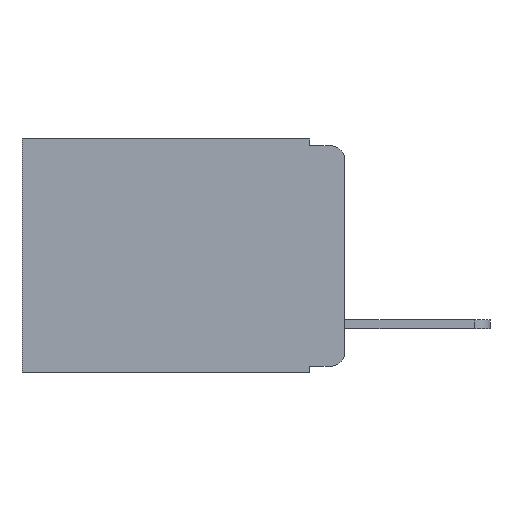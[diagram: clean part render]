
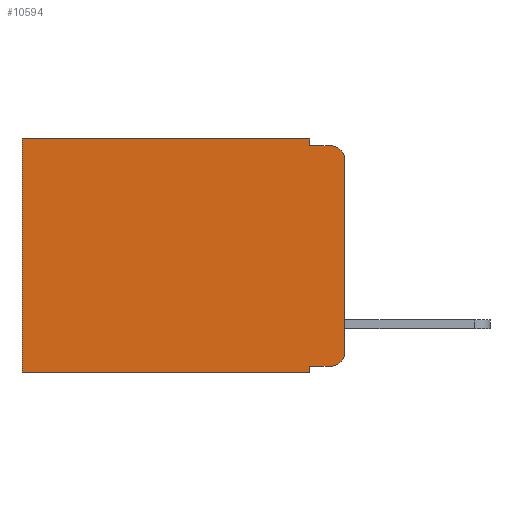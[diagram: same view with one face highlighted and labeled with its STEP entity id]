
A CAD part, left-side view. The second image highlights one B-rep face of the part: STEP entity #10594.
In plain terms, the highlighted planar face has unit normal (-1, 0, 0).
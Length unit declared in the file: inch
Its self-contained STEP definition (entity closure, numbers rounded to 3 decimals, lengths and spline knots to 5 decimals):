
#261 = AXIS2_PLACEMENT_3D ( 'NONE', #12687, #14218, #4974 ) ;
#318 = ORIENTED_EDGE ( 'NONE', *, *, #17588, .T. ) ;
#706 = DIRECTION ( 'NONE',  ( 0., 0., -1. ) ) ;
#741 = CARTESIAN_POINT ( 'NONE',  ( 0.298, 0., 0. ) ) ;
#1103 = VECTOR ( 'NONE', #18424, 39.37008 ) ;
#1160 = ORIENTED_EDGE ( 'NONE', *, *, #14528, .F. ) ;
#1178 = ORIENTED_EDGE ( 'NONE', *, *, #8918, .T. ) ;
#1285 = VERTEX_POINT ( 'NONE', #12991 ) ;
#1593 = VECTOR ( 'NONE', #1902, 39.37008 ) ;
#1785 = PLANE ( 'NONE',  #261 ) ;
#1902 = DIRECTION ( 'NONE',  ( 0., 0., -1. ) ) ;
#1999 = ORIENTED_EDGE ( 'NONE', *, *, #6705, .T. ) ;
#2133 = VECTOR ( 'NONE', #2357, 39.37008 ) ;
#2357 = DIRECTION ( 'NONE',  ( 0., 1., 0. ) ) ;
#2472 = LINE ( 'NONE', #14787, #13386 ) ;
#2897 = VECTOR ( 'NONE', #11029, 39.37008 ) ;
#3238 = CARTESIAN_POINT ( 'NONE',  ( 0.298, 0.02, -0.01 ) ) ;
#3276 = ORIENTED_EDGE ( 'NONE', *, *, #8655, .F. ) ;
#3520 = CARTESIAN_POINT ( 'NONE',  ( 0.298, 0.02, -0.333 ) ) ;
#3643 = CARTESIAN_POINT ( 'NONE',  ( 0.298, 0., -0.313 ) ) ;
#3924 = VERTEX_POINT ( 'NONE', #9028 ) ;
#3992 = CARTESIAN_POINT ( 'NONE',  ( 0.298, 0.473, 0. ) ) ;
#4182 = CARTESIAN_POINT ( 'NONE',  ( 0.298, 0.051, -0.333 ) ) ;
#4839 = CARTESIAN_POINT ( 'NONE',  ( 0.298, 0., -0.343 ) ) ;
#4880 = VERTEX_POINT ( 'NONE', #3520 ) ;
#4960 = ORIENTED_EDGE ( 'NONE', *, *, #11865, .F. ) ;
#4974 = DIRECTION ( 'NONE',  ( 0., 0., -1. ) ) ;
#5498 = DIRECTION ( 'NONE',  ( -1., 0., 0. ) ) ;
#5961 = ORIENTED_EDGE ( 'NONE', *, *, #12491, .T. ) ;
#6698 = CARTESIAN_POINT ( 'NONE',  ( 0.298, 0.051, 0. ) ) ;
#6705 = EDGE_CURVE ( 'NONE', #4880, #12149, #11502, .T. ) ;
#6712 = VECTOR ( 'NONE', #9175, 39.37008 ) ;
#6982 = VECTOR ( 'NONE', #16729, 39.37008 ) ;
#7832 = VERTEX_POINT ( 'NONE', #6698 ) ;
#8085 = CARTESIAN_POINT ( 'NONE',  ( 0.298, 0.051, -0.343 ) ) ;
#8186 = CARTESIAN_POINT ( 'NONE',  ( 0.298, 0.051, 0. ) ) ;
#8655 = EDGE_CURVE ( 'NONE', #13872, #3924, #18787, .T. ) ;
#8858 = ORIENTED_EDGE ( 'NONE', *, *, #16571, .F. ) ;
#8918 = EDGE_CURVE ( 'NONE', #7832, #10814, #10466, .T. ) ;
#9028 = CARTESIAN_POINT ( 'NONE',  ( 0.298, 0.473, -0.343 ) ) ;
#9175 = DIRECTION ( 'NONE',  ( 0., 0., -1. ) ) ;
#9807 = EDGE_CURVE ( 'NONE', #19686, #4880, #13509, .T. ) ;
#10140 = DIRECTION ( 'NONE',  ( -1., 0., 0. ) ) ;
#10250 = ORIENTED_EDGE ( 'NONE', *, *, #19611, .F. ) ;
#10466 = LINE ( 'NONE', #741, #2133 ) ;
#10504 = DIRECTION ( 'NONE',  ( 0., -1., 0. ) ) ;
#10594 = ADVANCED_FACE ( 'NONE', ( #14427 ), #1785, .F. ) ;
#10700 = CARTESIAN_POINT ( 'NONE',  ( 0.298, 0.051, 0. ) ) ;
#10706 = ORIENTED_EDGE ( 'NONE', *, *, #9807, .T. ) ;
#10814 = VERTEX_POINT ( 'NONE', #3992 ) ;
#10879 = VERTEX_POINT ( 'NONE', #15770 ) ;
#11000 = AXIS2_PLACEMENT_3D ( 'NONE', #14699, #5498, #16218 ) ;
#11029 = DIRECTION ( 'NONE',  ( 0., 1., 0. ) ) ;
#11078 = LINE ( 'NONE', #10700, #6982 ) ;
#11502 = CIRCLE ( 'NONE', #11000, 0.02 ) ;
#11582 = CIRCLE ( 'NONE', #15222, 0.02 ) ;
#11768 = LINE ( 'NONE', #19762, #6712 ) ;
#11865 = EDGE_CURVE ( 'NONE', #19686, #13872, #11078, .T. ) ;
#12149 = VERTEX_POINT ( 'NONE', #3643 ) ;
#12491 = EDGE_CURVE ( 'NONE', #10814, #3924, #11768, .T. ) ;
#12687 = CARTESIAN_POINT ( 'NONE',  ( 0.298, 0., 0. ) ) ;
#12991 = CARTESIAN_POINT ( 'NONE',  ( 0.298, 0.051, -0.01 ) ) ;
#13386 = VECTOR ( 'NONE', #17844, 39.37008 ) ;
#13509 = LINE ( 'NONE', #19881, #1103 ) ;
#13627 = CARTESIAN_POINT ( 'NONE',  ( 0.298, 0.051, -0.01 ) ) ;
#13872 = VERTEX_POINT ( 'NONE', #8085 ) ;
#13977 = EDGE_LOOP ( 'NONE', ( #10250, #318, #8858, #1160, #1178, #5961, #3276, #4960, #10706, #1999 ) ) ;
#14218 = DIRECTION ( 'NONE',  ( 1., 0., 0. ) ) ;
#14427 = FACE_OUTER_BOUND ( 'NONE', #13977, .T. ) ;
#14528 = EDGE_CURVE ( 'NONE', #7832, #1285, #18037, .T. ) ;
#14699 = CARTESIAN_POINT ( 'NONE',  ( 0.298, 0.02, -0.313 ) ) ;
#14787 = CARTESIAN_POINT ( 'NONE',  ( 0.298, 0., 0. ) ) ;
#15222 = AXIS2_PLACEMENT_3D ( 'NONE', #19217, #10140, #706 ) ;
#15323 = VECTOR ( 'NONE', #10504, 39.37008 ) ;
#15770 = CARTESIAN_POINT ( 'NONE',  ( 0.298, 0., -0.03 ) ) ;
#16218 = DIRECTION ( 'NONE',  ( 0., 0., -1. ) ) ;
#16571 = EDGE_CURVE ( 'NONE', #1285, #19312, #19357, .T. ) ;
#16729 = DIRECTION ( 'NONE',  ( 0., 0., -1. ) ) ;
#17588 = EDGE_CURVE ( 'NONE', #10879, #19312, #11582, .T. ) ;
#17844 = DIRECTION ( 'NONE',  ( 0., 0., -1. ) ) ;
#18037 = LINE ( 'NONE', #8186, #1593 ) ;
#18424 = DIRECTION ( 'NONE',  ( 0., -1., 0. ) ) ;
#18787 = LINE ( 'NONE', #4839, #2897 ) ;
#19217 = CARTESIAN_POINT ( 'NONE',  ( 0.298, 0.02, -0.03 ) ) ;
#19312 = VERTEX_POINT ( 'NONE', #3238 ) ;
#19357 = LINE ( 'NONE', #13627, #15323 ) ;
#19611 = EDGE_CURVE ( 'NONE', #10879, #12149, #2472, .T. ) ;
#19686 = VERTEX_POINT ( 'NONE', #4182 ) ;
#19762 = CARTESIAN_POINT ( 'NONE',  ( 0.298, 0.473, 0. ) ) ;
#19881 = CARTESIAN_POINT ( 'NONE',  ( 0.298, 0.051, -0.333 ) ) ;
